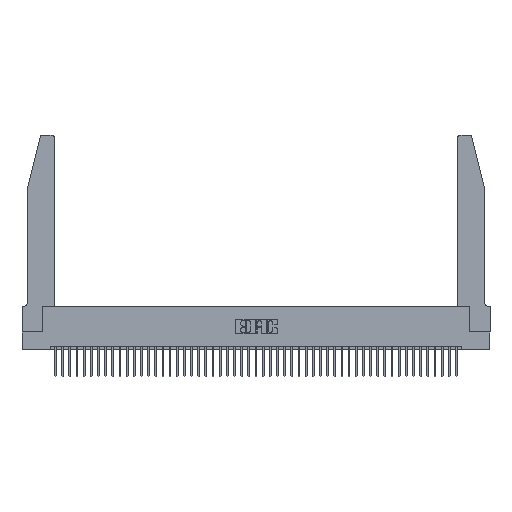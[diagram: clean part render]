
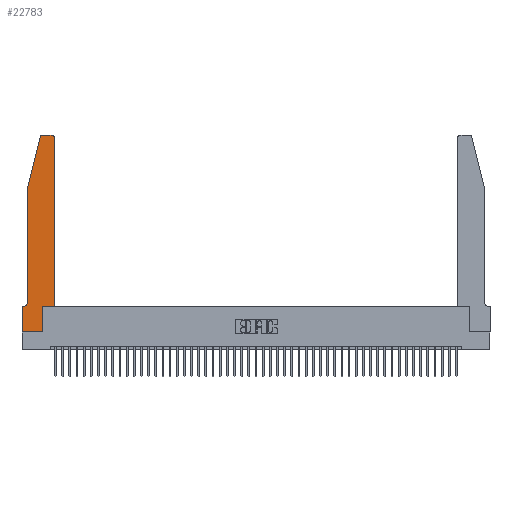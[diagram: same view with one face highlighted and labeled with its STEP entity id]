
A CAD part, top view. The second image highlights one B-rep face of the part: STEP entity #22783.
In plain terms, the highlighted planar face has unit normal (0, 0, 1).
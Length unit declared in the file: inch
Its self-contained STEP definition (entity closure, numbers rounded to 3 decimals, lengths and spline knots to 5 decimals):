
#39 = VECTOR ( 'NONE', #31280, 39.37008 ) ;
#1656 = LINE ( 'NONE', #24234, #14349 ) ;
#1843 = EDGE_CURVE ( 'NONE', #28759, #10305, #32569, .T. ) ;
#1869 = CIRCLE ( 'NONE', #25334, 0.03 ) ;
#2462 = VERTEX_POINT ( 'NONE', #16671 ) ;
#2842 = FACE_OUTER_BOUND ( 'NONE', #9192, .T. ) ;
#2900 = VERTEX_POINT ( 'NONE', #18054 ) ;
#3795 = ORIENTED_EDGE ( 'NONE', *, *, #17669, .T. ) ;
#4943 = AXIS2_PLACEMENT_3D ( 'NONE', #20494, #21436, #17275 ) ;
#4990 = ORIENTED_EDGE ( 'NONE', *, *, #42389, .T. ) ;
#5187 = DIRECTION ( 'NONE',  ( 0., 1., 0. ) ) ;
#6588 = DIRECTION ( 'NONE',  ( -1., 0., 0. ) ) ;
#6743 = CARTESIAN_POINT ( 'NONE',  ( 0.0755, 2., 0.37 ) ) ;
#7107 = CARTESIAN_POINT ( 'NONE',  ( 0.0755, 0.35, 0.37 ) ) ;
#9192 = EDGE_LOOP ( 'NONE', ( #25023, #46753, #42508, #29073, #4990, #9569, #23179, #18077, #27168, #31345, #3795, #47111 ) ) ;
#9276 = CARTESIAN_POINT ( 'NONE',  ( 0.4505, 0.35, 0.37 ) ) ;
#9453 = CARTESIAN_POINT ( 'NONE',  ( 0.0055, 0.42, 0.37 ) ) ;
#9569 = ORIENTED_EDGE ( 'NONE', *, *, #1843, .T. ) ;
#10024 = LINE ( 'NONE', #46972, #27174 ) ;
#10225 = VECTOR ( 'NONE', #5187, 39.37008 ) ;
#10305 = VERTEX_POINT ( 'NONE', #15173 ) ;
#10316 = EDGE_CURVE ( 'NONE', #36640, #47191, #45258, .T. ) ;
#10781 = VECTOR ( 'NONE', #39202, 39.37008 ) ;
#10784 = VECTOR ( 'NONE', #47186, 39.37008 ) ;
#11154 = LINE ( 'NONE', #21769, #42113 ) ;
#12829 = CARTESIAN_POINT ( 'NONE',  ( 0.4505, 0.35, 0.37 ) ) ;
#13113 = PLANE ( 'NONE',  #4943 ) ;
#13151 = DIRECTION ( 'NONE',  ( 0., -1., 0. ) ) ;
#14132 = DIRECTION ( 'NONE',  ( 0., -1., 0. ) ) ;
#14349 = VECTOR ( 'NONE', #13151, 39.37008 ) ;
#15173 = CARTESIAN_POINT ( 'NONE',  ( 0., 0.35, 0.37 ) ) ;
#15318 = EDGE_CURVE ( 'NONE', #19917, #2462, #47254, .T. ) ;
#16671 = CARTESIAN_POINT ( 'NONE',  ( 0.2865, 0., 0.37 ) ) ;
#17275 = DIRECTION ( 'NONE',  ( 1., 0., 0. ) ) ;
#17425 = CARTESIAN_POINT ( 'NONE',  ( 0.2865, 0.35, 0.37 ) ) ;
#17669 = EDGE_CURVE ( 'NONE', #20814, #40730, #39052, .T. ) ;
#17715 = DIRECTION ( 'NONE',  ( 0., 0., 1. ) ) ;
#18054 = CARTESIAN_POINT ( 'NONE',  ( 0.0755, 2., 0.37 ) ) ;
#18077 = ORIENTED_EDGE ( 'NONE', *, *, #15318, .T. ) ;
#19343 = CARTESIAN_POINT ( 'NONE',  ( 0., 0., 0.37 ) ) ;
#19459 = DIRECTION ( 'NONE',  ( 1., 0., 0. ) ) ;
#19917 = VERTEX_POINT ( 'NONE', #19343 ) ;
#20315 = CARTESIAN_POINT ( 'NONE',  ( 0.284, 2.72, 0.37 ) ) ;
#20461 = CARTESIAN_POINT ( 'NONE',  ( 0.0755, 2., 0.37 ) ) ;
#20494 = CARTESIAN_POINT ( 'NONE',  ( 0., 0.35, 0.37 ) ) ;
#20503 = LINE ( 'NONE', #26636, #10225 ) ;
#20515 = LINE ( 'NONE', #20461, #10781 ) ;
#20784 = DIRECTION ( 'NONE',  ( 1., 0., 0. ) ) ;
#20814 = VERTEX_POINT ( 'NONE', #9276 ) ;
#21436 = DIRECTION ( 'NONE',  ( 0., 0., 1. ) ) ;
#21769 = CARTESIAN_POINT ( 'NONE',  ( 0.4505, 0.35, 0.37 ) ) ;
#21841 = DIRECTION ( 'NONE',  ( 1., 0., 0. ) ) ;
#22783 = ADVANCED_FACE ( 'NONE', ( #2842 ), #13113, .T. ) ;
#23179 = ORIENTED_EDGE ( 'NONE', *, *, #36887, .T. ) ;
#23231 = EDGE_CURVE ( 'NONE', #2900, #46520, #46402, .T. ) ;
#24234 = CARTESIAN_POINT ( 'NONE',  ( 0., 0., 0.37 ) ) ;
#25023 = ORIENTED_EDGE ( 'NONE', *, *, #34333, .T. ) ;
#25334 = AXIS2_PLACEMENT_3D ( 'NONE', #28774, #17715, #36919 ) ;
#26636 = CARTESIAN_POINT ( 'NONE',  ( 0.2865, 0.35, 0.37 ) ) ;
#27168 = ORIENTED_EDGE ( 'NONE', *, *, #38009, .T. ) ;
#27174 = VECTOR ( 'NONE', #6588, 39.37008 ) ;
#27728 = VECTOR ( 'NONE', #21841, 39.37008 ) ;
#28759 = VERTEX_POINT ( 'NONE', #35417 ) ;
#28774 = CARTESIAN_POINT ( 'NONE',  ( 0.4205, 2.72, 0.37 ) ) ;
#29073 = ORIENTED_EDGE ( 'NONE', *, *, #23231, .T. ) ;
#29341 = CARTESIAN_POINT ( 'NONE',  ( 0., 0., 0.37 ) ) ;
#29649 = CARTESIAN_POINT ( 'NONE',  ( 0.4205, 2.75, 0.37 ) ) ;
#29758 = AXIS2_PLACEMENT_3D ( 'NONE', #20315, #31707, #20784 ) ;
#30727 = EDGE_CURVE ( 'NONE', #47191, #2900, #20515, .T. ) ;
#31280 = DIRECTION ( 'NONE',  ( 0., 1., 0. ) ) ;
#31345 = ORIENTED_EDGE ( 'NONE', *, *, #34536, .T. ) ;
#31707 = DIRECTION ( 'NONE',  ( 0., 0., 1. ) ) ;
#31881 = DIRECTION ( 'NONE',  ( 0., 0., -1. ) ) ;
#32569 = LINE ( 'NONE', #7107, #10784 ) ;
#33495 = CARTESIAN_POINT ( 'NONE',  ( 0.284, 2.75, 0.37 ) ) ;
#34333 = EDGE_CURVE ( 'NONE', #46856, #36640, #10024, .T. ) ;
#34536 = EDGE_CURVE ( 'NONE', #45963, #20814, #11154, .T. ) ;
#35023 = EDGE_CURVE ( 'NONE', #40730, #46856, #1869, .T. ) ;
#35380 = DIRECTION ( 'NONE',  ( -1., 0., 0. ) ) ;
#35417 = CARTESIAN_POINT ( 'NONE',  ( 0.0055, 0.35, 0.37 ) ) ;
#36640 = VERTEX_POINT ( 'NONE', #33495 ) ;
#36887 = EDGE_CURVE ( 'NONE', #10305, #19917, #1656, .T. ) ;
#36919 = DIRECTION ( 'NONE',  ( 1., 0., 0. ) ) ;
#38009 = EDGE_CURVE ( 'NONE', #2462, #45963, #20503, .T. ) ;
#38366 = AXIS2_PLACEMENT_3D ( 'NONE', #9453, #31881, #35380 ) ;
#39052 = LINE ( 'NONE', #12829, #39 ) ;
#39202 = DIRECTION ( 'NONE',  ( -0.239, -0.971, 0. ) ) ;
#40025 = CARTESIAN_POINT ( 'NONE',  ( 0.4505, 2.72, 0.37 ) ) ;
#40730 = VERTEX_POINT ( 'NONE', #40025 ) ;
#41767 = VECTOR ( 'NONE', #14132, 39.37008 ) ;
#42066 = CARTESIAN_POINT ( 'NONE',  ( 0.0755, 0.42, 0.37 ) ) ;
#42113 = VECTOR ( 'NONE', #19459, 39.37008 ) ;
#42389 = EDGE_CURVE ( 'NONE', #46520, #28759, #43503, .T. ) ;
#42508 = ORIENTED_EDGE ( 'NONE', *, *, #30727, .T. ) ;
#43503 = CIRCLE ( 'NONE', #38366, 0.07 ) ;
#45258 = CIRCLE ( 'NONE', #29758, 0.03 ) ;
#45963 = VERTEX_POINT ( 'NONE', #17425 ) ;
#46402 = LINE ( 'NONE', #6743, #41767 ) ;
#46520 = VERTEX_POINT ( 'NONE', #42066 ) ;
#46753 = ORIENTED_EDGE ( 'NONE', *, *, #10316, .T. ) ;
#46850 = CARTESIAN_POINT ( 'NONE',  ( 0.25487, 2.72718, 0.37 ) ) ;
#46856 = VERTEX_POINT ( 'NONE', #29649 ) ;
#46972 = CARTESIAN_POINT ( 'NONE',  ( 0.2605, 2.75, 0.37 ) ) ;
#47111 = ORIENTED_EDGE ( 'NONE', *, *, #35023, .T. ) ;
#47186 = DIRECTION ( 'NONE',  ( -1., 0., 0. ) ) ;
#47191 = VERTEX_POINT ( 'NONE', #46850 ) ;
#47254 = LINE ( 'NONE', #29341, #27728 ) ;
